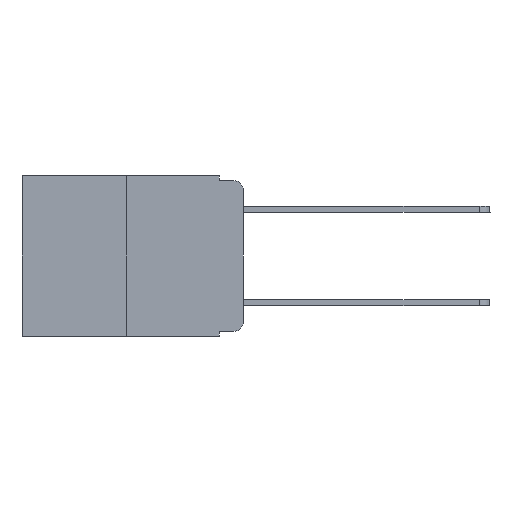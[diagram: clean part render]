
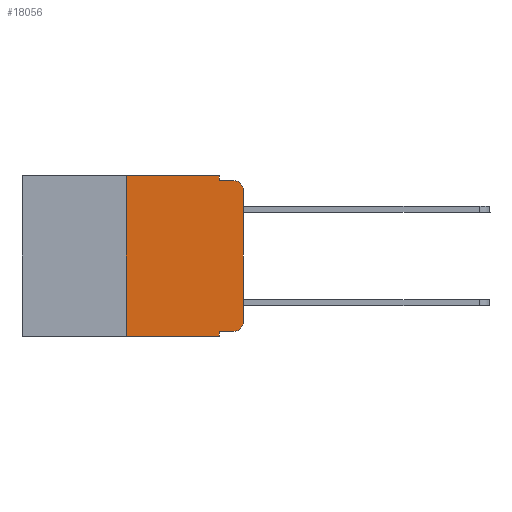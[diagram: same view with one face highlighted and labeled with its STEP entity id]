
A CAD part, left-side view. The second image highlights one B-rep face of the part: STEP entity #18056.
In plain terms, the highlighted planar face has unit normal (-1, 0, 0).
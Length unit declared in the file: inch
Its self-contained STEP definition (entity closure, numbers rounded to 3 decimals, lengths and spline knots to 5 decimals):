
#299 = ORIENTED_EDGE ( 'NONE', *, *, #24387, .T. ) ;
#354 = EDGE_CURVE ( 'NONE', #3922, #15330, #13289, .T. ) ;
#361 = VECTOR ( 'NONE', #15045, 39.37008 ) ;
#523 = VERTEX_POINT ( 'NONE', #11677 ) ;
#708 = LINE ( 'NONE', #13925, #9794 ) ;
#866 = ORIENTED_EDGE ( 'NONE', *, *, #18615, .T. ) ;
#978 = CARTESIAN_POINT ( 'NONE',  ( 0., 0.02, -0.333 ) ) ;
#2008 = CARTESIAN_POINT ( 'NONE',  ( 0., 0.02, -0.01 ) ) ;
#2163 = VERTEX_POINT ( 'NONE', #978 ) ;
#2166 = EDGE_CURVE ( 'NONE', #12415, #24555, #4975, .T. ) ;
#3214 = VERTEX_POINT ( 'NONE', #14422 ) ;
#3535 = CARTESIAN_POINT ( 'NONE',  ( 0., 0., 0. ) ) ;
#3539 = EDGE_CURVE ( 'NONE', #10689, #22587, #24000, .T. ) ;
#3687 = CARTESIAN_POINT ( 'NONE',  ( 0., 0.473, -0.343 ) ) ;
#3863 = EDGE_CURVE ( 'NONE', #4582, #22587, #9141, .T. ) ;
#3922 = VERTEX_POINT ( 'NONE', #3941 ) ;
#3941 = CARTESIAN_POINT ( 'NONE',  ( 0., 0.051, -0.01 ) ) ;
#4270 = DIRECTION ( 'NONE',  ( 0., -1., 0. ) ) ;
#4582 = VERTEX_POINT ( 'NONE', #11138 ) ;
#4958 = DIRECTION ( 'NONE',  ( 0., 0., -1. ) ) ;
#4975 = LINE ( 'NONE', #14672, #11364 ) ;
#5586 = DIRECTION ( 'NONE',  ( 0., -1., 0. ) ) ;
#6139 = ORIENTED_EDGE ( 'NONE', *, *, #3539, .F. ) ;
#7006 = ORIENTED_EDGE ( 'NONE', *, *, #14947, .F. ) ;
#7292 = CARTESIAN_POINT ( 'NONE',  ( 0., 0.051, 0. ) ) ;
#7330 = VECTOR ( 'NONE', #17222, 39.37008 ) ;
#7345 = CARTESIAN_POINT ( 'NONE',  ( 0., 0.051, -0.333 ) ) ;
#7493 = EDGE_CURVE ( 'NONE', #4582, #12415, #23538, .T. ) ;
#8077 = DIRECTION ( 'NONE',  ( 0., 0., -1. ) ) ;
#8409 = CARTESIAN_POINT ( 'NONE',  ( 0., 0.25, 0. ) ) ;
#9039 = VECTOR ( 'NONE', #5586, 39.37008 ) ;
#9141 = LINE ( 'NONE', #3687, #7330 ) ;
#9215 = CIRCLE ( 'NONE', #23841, 0.02 ) ;
#9432 = EDGE_LOOP ( 'NONE', ( #299, #17360, #19779, #7006, #23547, #15402, #16437, #6139, #10171, #866 ) ) ;
#9794 = VECTOR ( 'NONE', #4270, 39.37008 ) ;
#10053 = CARTESIAN_POINT ( 'NONE',  ( 0., 0.02, -0.03 ) ) ;
#10171 = ORIENTED_EDGE ( 'NONE', *, *, #10458, .T. ) ;
#10377 = EDGE_CURVE ( 'NONE', #523, #15330, #9215, .T. ) ;
#10458 = EDGE_CURVE ( 'NONE', #10689, #2163, #708, .T. ) ;
#10555 = DIRECTION ( 'NONE',  ( 0., -1., 0. ) ) ;
#10689 = VERTEX_POINT ( 'NONE', #7345 ) ;
#11138 = CARTESIAN_POINT ( 'NONE',  ( 0., 0.25, -0.343 ) ) ;
#11364 = VECTOR ( 'NONE', #10555, 39.37008 ) ;
#11677 = CARTESIAN_POINT ( 'NONE',  ( 0., 0., -0.03 ) ) ;
#12415 = VERTEX_POINT ( 'NONE', #14263 ) ;
#12763 = PLANE ( 'NONE',  #15503 ) ;
#13289 = LINE ( 'NONE', #16119, #9039 ) ;
#13844 = DIRECTION ( 'NONE',  ( -1., 0., 0. ) ) ;
#13925 = CARTESIAN_POINT ( 'NONE',  ( 0., 0.051, -0.333 ) ) ;
#14263 = CARTESIAN_POINT ( 'NONE',  ( 0., 0.25, 0. ) ) ;
#14340 = CARTESIAN_POINT ( 'NONE',  ( 0., 0.051, 0. ) ) ;
#14422 = CARTESIAN_POINT ( 'NONE',  ( 0., 0., -0.313 ) ) ;
#14601 = DIRECTION ( 'NONE',  ( 1., 0., 0. ) ) ;
#14672 = CARTESIAN_POINT ( 'NONE',  ( 0., 0.473, 0. ) ) ;
#14947 = EDGE_CURVE ( 'NONE', #24555, #3922, #17131, .T. ) ;
#15045 = DIRECTION ( 'NONE',  ( 0., 0., -1. ) ) ;
#15149 = CIRCLE ( 'NONE', #17754, 0.02 ) ;
#15330 = VERTEX_POINT ( 'NONE', #2008 ) ;
#15402 = ORIENTED_EDGE ( 'NONE', *, *, #7493, .F. ) ;
#15503 = AXIS2_PLACEMENT_3D ( 'NONE', #24528, #14601, #4958 ) ;
#15925 = DIRECTION ( 'NONE',  ( 0., 0., 1. ) ) ;
#16119 = CARTESIAN_POINT ( 'NONE',  ( 0., 0.051, -0.01 ) ) ;
#16437 = ORIENTED_EDGE ( 'NONE', *, *, #3863, .T. ) ;
#16642 = DIRECTION ( 'NONE',  ( 0., 0., -1. ) ) ;
#16824 = VECTOR ( 'NONE', #16642, 39.37008 ) ;
#17064 = DIRECTION ( 'NONE',  ( 0., 0., 1. ) ) ;
#17131 = LINE ( 'NONE', #20368, #16824 ) ;
#17222 = DIRECTION ( 'NONE',  ( 0., -1., 0. ) ) ;
#17360 = ORIENTED_EDGE ( 'NONE', *, *, #10377, .T. ) ;
#17400 = CARTESIAN_POINT ( 'NONE',  ( 0., 0.051, -0.343 ) ) ;
#17456 = VECTOR ( 'NONE', #15925, 39.37008 ) ;
#17754 = AXIS2_PLACEMENT_3D ( 'NONE', #17860, #19663, #8077 ) ;
#17860 = CARTESIAN_POINT ( 'NONE',  ( 0., 0.02, -0.313 ) ) ;
#18039 = DIRECTION ( 'NONE',  ( 0., 0., -1. ) ) ;
#18056 = ADVANCED_FACE ( 'NONE', ( #22482 ), #12763, .F. ) ;
#18453 = LINE ( 'NONE', #3535, #21529 ) ;
#18615 = EDGE_CURVE ( 'NONE', #2163, #3214, #15149, .T. ) ;
#19663 = DIRECTION ( 'NONE',  ( -1., 0., 0. ) ) ;
#19779 = ORIENTED_EDGE ( 'NONE', *, *, #354, .F. ) ;
#20368 = CARTESIAN_POINT ( 'NONE',  ( 0., 0.051, 0. ) ) ;
#21529 = VECTOR ( 'NONE', #17064, 39.37008 ) ;
#22482 = FACE_OUTER_BOUND ( 'NONE', #9432, .T. ) ;
#22587 = VERTEX_POINT ( 'NONE', #17400 ) ;
#23538 = LINE ( 'NONE', #8409, #17456 ) ;
#23547 = ORIENTED_EDGE ( 'NONE', *, *, #2166, .F. ) ;
#23841 = AXIS2_PLACEMENT_3D ( 'NONE', #10053, #13844, #18039 ) ;
#24000 = LINE ( 'NONE', #7292, #361 ) ;
#24387 = EDGE_CURVE ( 'NONE', #3214, #523, #18453, .T. ) ;
#24528 = CARTESIAN_POINT ( 'NONE',  ( 0., 0.473, 0. ) ) ;
#24555 = VERTEX_POINT ( 'NONE', #14340 ) ;
